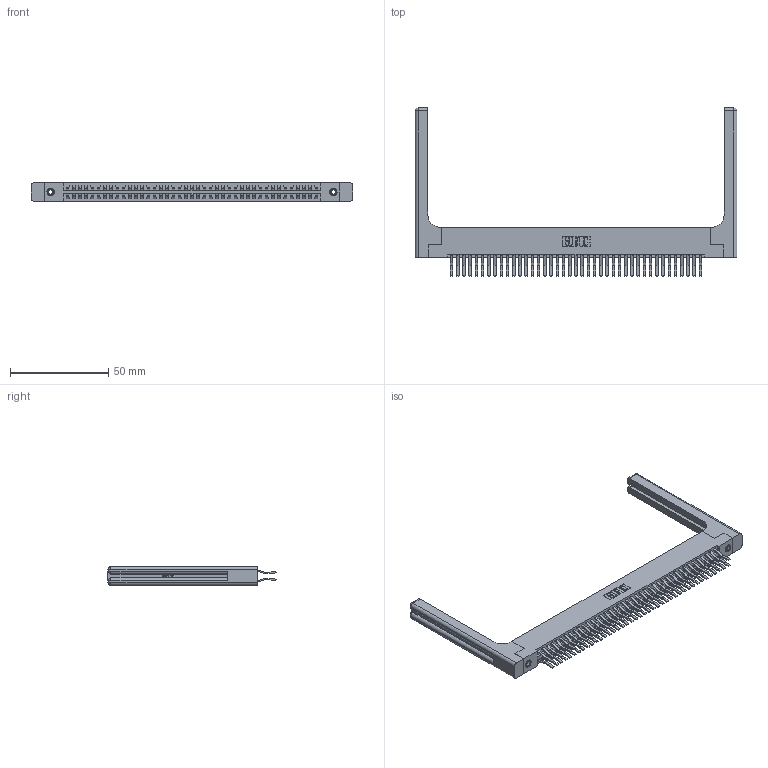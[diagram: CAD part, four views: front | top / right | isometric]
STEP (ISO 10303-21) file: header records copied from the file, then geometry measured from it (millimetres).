
FILE_DESCRIPTION (( 'STEP AP203' ), '1' );
FILE_NAME ('396-082-560-258.STEP', '2019-10-30T23:45:23', ( '' ), ( '' ), 'SwSTEP 2.0', 'SolidWorks 2016', '' );
FILE_SCHEMA (( 'CONFIG_CONTROL_DESIGN' ));
Length unit declared in the file: inch
Products named in the file (5): 346 Part_Flush Mounting Lugs - 0.156 Dia-TH; 346-220-058_345-220-058; 396-082-560-258; 345-292-001_560 Tail; 345-250-001_345-250-001-102
Assembly tree (87 placements, depth 2):
  396-082-560-258
    346 Part_Flush Mounting Lugs - 0.156 Dia-TH
    345-292-001_560 Tail  x82
    345-250-001_345-250-001-102  x2
    346-220-058_345-220-058  x2
Bounding box: 164.24 x 85.74 x 9.4 mm (x, y, z)
Volume: 24039 mm3; surface area: 29133 mm2
Topology: 87 solids, 87 shells, 4806 faces, 14197 edges, 9334 vertices
Faces by surface type: plane 3094, cylinder 1652, bspline 36, cone 12, sphere 8, torus 4
Entity records: 32162 total; most frequent: CARTESIAN_POINT 6309, ORIENTED_EDGE 5040, DIRECTION 4548, EDGE_CURVE 2520, LINE 2128, VECTOR 2128, VERTEX_POINT 1670, AXIS2_PLACEMENT_3D 1210
